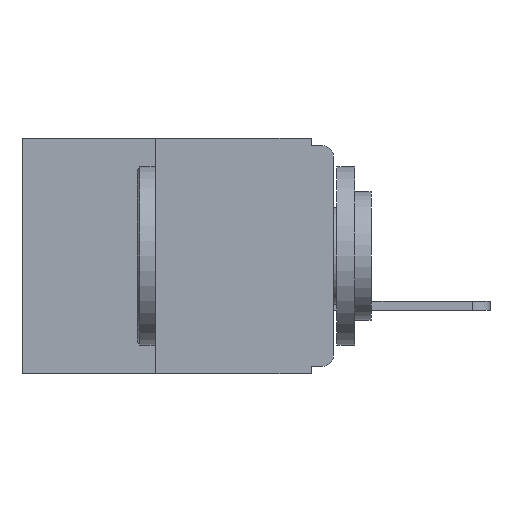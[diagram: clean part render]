
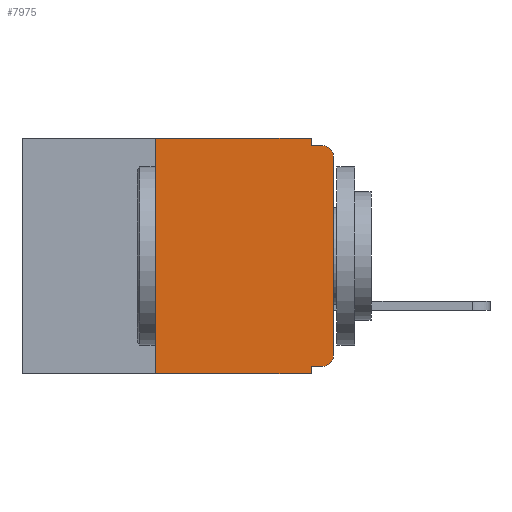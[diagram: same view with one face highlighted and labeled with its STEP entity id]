
A CAD part, left-side view. The second image highlights one B-rep face of the part: STEP entity #7975.
In plain terms, the highlighted planar face has unit normal (-1, 0, 0).
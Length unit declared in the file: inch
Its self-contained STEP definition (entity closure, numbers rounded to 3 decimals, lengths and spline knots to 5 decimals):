
#786 = DIRECTION ( 'NONE',  ( 0., 0., -1. ) ) ;
#1355 = VERTEX_POINT ( 'NONE', #17011 ) ;
#2624 = DIRECTION ( 'NONE',  ( 0., 0., -1. ) ) ;
#2698 = DIRECTION ( 'NONE',  ( 1., 0., 0. ) ) ;
#2809 = EDGE_CURVE ( 'NONE', #20911, #3972, #13266, .T. ) ;
#2873 = CARTESIAN_POINT ( 'NONE',  ( 0., 0.437, 0. ) ) ;
#2931 = PLANE ( 'NONE',  #7615 ) ;
#2957 = CARTESIAN_POINT ( 'NONE',  ( 0., 0.031, -0.33 ) ) ;
#3121 = LINE ( 'NONE', #20299, #16234 ) ;
#3279 = ORIENTED_EDGE ( 'NONE', *, *, #23236, .T. ) ;
#3972 = VERTEX_POINT ( 'NONE', #26433 ) ;
#4345 = EDGE_CURVE ( 'NONE', #3972, #1355, #3121, .T. ) ;
#4391 = VECTOR ( 'NONE', #11954, 39.37008 ) ;
#4499 = VERTEX_POINT ( 'NONE', #16874 ) ;
#5303 = DIRECTION ( 'NONE',  ( -1., 0., 0. ) ) ;
#7597 = CARTESIAN_POINT ( 'NONE',  ( 0., 0.015, -0.01 ) ) ;
#7615 = AXIS2_PLACEMENT_3D ( 'NONE', #2873, #2698, #2624 ) ;
#7695 = EDGE_CURVE ( 'NONE', #23069, #20911, #17573, .T. ) ;
#7862 = DIRECTION ( 'NONE',  ( 0., 0., 1. ) ) ;
#7975 = ADVANCED_FACE ( 'NONE', ( #27902 ), #2931, .F. ) ;
#8162 = CARTESIAN_POINT ( 'NONE',  ( 0., 0.25, -0.33 ) ) ;
#8902 = VECTOR ( 'NONE', #15637, 39.37008 ) ;
#9421 = CARTESIAN_POINT ( 'NONE',  ( 0., 0.015, -0.32 ) ) ;
#9782 = LINE ( 'NONE', #9992, #27817 ) ;
#9992 = CARTESIAN_POINT ( 'NONE',  ( 0., 0., -0.01 ) ) ;
#10086 = DIRECTION ( 'NONE',  ( 0., 0., 1. ) ) ;
#10148 = CARTESIAN_POINT ( 'NONE',  ( 0., 0.25, -0.33 ) ) ;
#10237 = ORIENTED_EDGE ( 'NONE', *, *, #27107, .F. ) ;
#10419 = VERTEX_POINT ( 'NONE', #9421 ) ;
#10578 = EDGE_CURVE ( 'NONE', #10419, #10950, #27919, .T. ) ;
#10607 = ORIENTED_EDGE ( 'NONE', *, *, #22023, .T. ) ;
#10950 = VERTEX_POINT ( 'NONE', #24096 ) ;
#11788 = VECTOR ( 'NONE', #14350, 39.37008 ) ;
#11873 = CARTESIAN_POINT ( 'NONE',  ( 0., 0., -0.32 ) ) ;
#11954 = DIRECTION ( 'NONE',  ( 0., -1., 0. ) ) ;
#12502 = DIRECTION ( 'NONE',  ( 0., -1., 0. ) ) ;
#12862 = AXIS2_PLACEMENT_3D ( 'NONE', #20051, #5303, #22526 ) ;
#13266 = LINE ( 'NONE', #21788, #4391 ) ;
#13345 = LINE ( 'NONE', #11873, #11788 ) ;
#14137 = LINE ( 'NONE', #2957, #26399 ) ;
#14350 = DIRECTION ( 'NONE',  ( 0., 1., 0. ) ) ;
#15426 = VERTEX_POINT ( 'NONE', #19001 ) ;
#15472 = DIRECTION ( 'NONE',  ( -1., 0., 0. ) ) ;
#15637 = DIRECTION ( 'NONE',  ( 0., -1., 0. ) ) ;
#15728 = VERTEX_POINT ( 'NONE', #28086 ) ;
#16020 = ORIENTED_EDGE ( 'NONE', *, *, #23179, .T. ) ;
#16056 = EDGE_LOOP ( 'NONE', ( #3279, #10607, #17153, #18679, #25202, #27502, #16020, #10237, #29441, #17184 ) ) ;
#16234 = VECTOR ( 'NONE', #20557, 39.37008 ) ;
#16874 = CARTESIAN_POINT ( 'NONE',  ( 0., 0.031, -0.32 ) ) ;
#17011 = CARTESIAN_POINT ( 'NONE',  ( 0., 0.031, -0.01 ) ) ;
#17153 = ORIENTED_EDGE ( 'NONE', *, *, #21908, .F. ) ;
#17184 = ORIENTED_EDGE ( 'NONE', *, *, #10578, .T. ) ;
#17404 = AXIS2_PLACEMENT_3D ( 'NONE', #30149, #15472, #786 ) ;
#17573 = LINE ( 'NONE', #8162, #22581 ) ;
#17673 = DIRECTION ( 'NONE',  ( 0., 0., -1. ) ) ;
#18679 = ORIENTED_EDGE ( 'NONE', *, *, #4345, .F. ) ;
#19001 = CARTESIAN_POINT ( 'NONE',  ( 0., 0., -0.025 ) ) ;
#20051 = CARTESIAN_POINT ( 'NONE',  ( 0., 0.015, -0.305 ) ) ;
#20299 = CARTESIAN_POINT ( 'NONE',  ( 0., 0.031, 0. ) ) ;
#20557 = DIRECTION ( 'NONE',  ( 0., 0., -1. ) ) ;
#20625 = VERTEX_POINT ( 'NONE', #7597 ) ;
#20911 = VERTEX_POINT ( 'NONE', #26028 ) ;
#21035 = EDGE_CURVE ( 'NONE', #10419, #4499, #13345, .T. ) ;
#21204 = VECTOR ( 'NONE', #10086, 39.37008 ) ;
#21788 = CARTESIAN_POINT ( 'NONE',  ( 0., 0.437, 0. ) ) ;
#21908 = EDGE_CURVE ( 'NONE', #1355, #20625, #9782, .T. ) ;
#22023 = EDGE_CURVE ( 'NONE', #15426, #20625, #24745, .T. ) ;
#22344 = CARTESIAN_POINT ( 'NONE',  ( 0., 0., 0. ) ) ;
#22526 = DIRECTION ( 'NONE',  ( 0., 0., -1. ) ) ;
#22581 = VECTOR ( 'NONE', #7862, 39.37008 ) ;
#23069 = VERTEX_POINT ( 'NONE', #10148 ) ;
#23179 = EDGE_CURVE ( 'NONE', #23069, #15728, #28492, .T. ) ;
#23236 = EDGE_CURVE ( 'NONE', #10950, #15426, #26959, .T. ) ;
#24096 = CARTESIAN_POINT ( 'NONE',  ( 0., 0., -0.305 ) ) ;
#24745 = CIRCLE ( 'NONE', #17404, 0.015 ) ;
#25202 = ORIENTED_EDGE ( 'NONE', *, *, #2809, .F. ) ;
#26028 = CARTESIAN_POINT ( 'NONE',  ( 0., 0.25, 0. ) ) ;
#26399 = VECTOR ( 'NONE', #17673, 39.37008 ) ;
#26433 = CARTESIAN_POINT ( 'NONE',  ( 0., 0.031, 0. ) ) ;
#26959 = LINE ( 'NONE', #22344, #21204 ) ;
#27107 = EDGE_CURVE ( 'NONE', #4499, #15728, #14137, .T. ) ;
#27502 = ORIENTED_EDGE ( 'NONE', *, *, #7695, .F. ) ;
#27817 = VECTOR ( 'NONE', #12502, 39.37008 ) ;
#27831 = CARTESIAN_POINT ( 'NONE',  ( 0., 0.437, -0.33 ) ) ;
#27902 = FACE_OUTER_BOUND ( 'NONE', #16056, .T. ) ;
#27919 = CIRCLE ( 'NONE', #12862, 0.015 ) ;
#28086 = CARTESIAN_POINT ( 'NONE',  ( 0., 0.031, -0.33 ) ) ;
#28492 = LINE ( 'NONE', #27831, #8902 ) ;
#29441 = ORIENTED_EDGE ( 'NONE', *, *, #21035, .F. ) ;
#30149 = CARTESIAN_POINT ( 'NONE',  ( 0., 0.015, -0.025 ) ) ;
